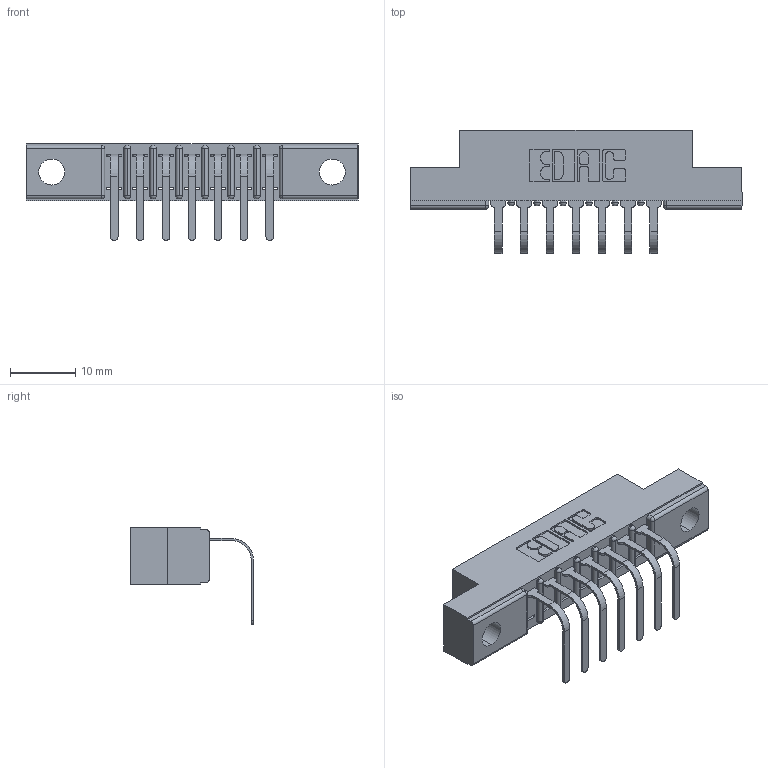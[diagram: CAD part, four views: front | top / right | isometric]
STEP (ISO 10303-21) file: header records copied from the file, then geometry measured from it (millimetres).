
FILE_DESCRIPTION (( 'STEP AP203' ), '1' );
FILE_NAME ('357-007-558-102.STEP', '2022-07-13T22:49:08', ( '' ), ( '' ), 'SwSTEP 2.0', 'SolidWorks 2020', '' );
FILE_SCHEMA (( 'CONFIG_CONTROL_DESIGN' ));
Length unit declared in the file: inch
Products named in the file (3): 307 Part_.128 Dia Mounting Holes; 357-007-558-102; 307-290-001_558 - 2 (Single)
Assembly tree (8 placements, depth 2):
  357-007-558-102
    307 Part_.128 Dia Mounting Holes
    307-290-001_558 - 2 (Single)  x7
Bounding box: 50.75 x 18.78 x 14.81 mm (x, y, z)
Volume: 3182.5 mm3; surface area: 4377.2 mm2
Topology: 8 solids, 8 shells, 546 faces, 1541 edges, 994 vertices
Faces by surface type: plane 343, cylinder 187, sphere 16
Entity records: 10422 total; most frequent: CARTESIAN_POINT 1744, ORIENTED_EDGE 1730, DIRECTION 1717, EDGE_CURVE 865, LINE 647, VECTOR 647, VERTEX_POINT 562, AXIS2_PLACEMENT_3D 535
